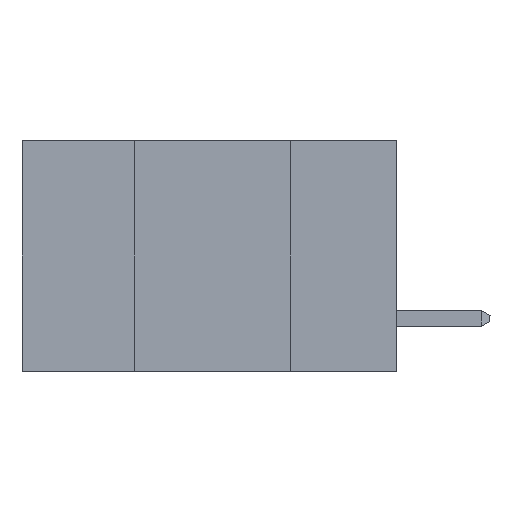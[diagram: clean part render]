
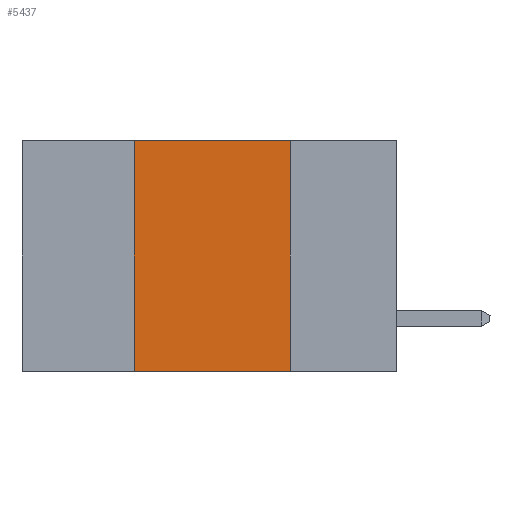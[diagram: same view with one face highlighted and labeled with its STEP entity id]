
A CAD part, left-side view. The second image highlights one B-rep face of the part: STEP entity #5437.
In plain terms, the highlighted planar face has unit normal (-1, 0, 0).
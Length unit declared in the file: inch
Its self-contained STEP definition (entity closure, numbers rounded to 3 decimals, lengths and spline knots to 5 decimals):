
#397 = LINE ( 'NONE', #22797, #23867 ) ;
#603 = DIRECTION ( 'NONE',  ( 0., 0., -1. ) ) ;
#2635 = ORIENTED_EDGE ( 'NONE', *, *, #13744, .F. ) ;
#4188 = LINE ( 'NONE', #6854, #21523 ) ;
#5243 = FACE_OUTER_BOUND ( 'NONE', #16323, .T. ) ;
#5365 = VERTEX_POINT ( 'NONE', #11476 ) ;
#5437 = ADVANCED_FACE ( 'NONE', ( #5243 ), #13830, .F. ) ;
#6231 = DIRECTION ( 'NONE',  ( 0., 0., -1. ) ) ;
#6854 = CARTESIAN_POINT ( 'NONE',  ( 0., 0.6, -0.37 ) ) ;
#8241 = EDGE_CURVE ( 'NONE', #13775, #5365, #397, .T. ) ;
#9029 = VECTOR ( 'NONE', #19841, 39.37008 ) ;
#9602 = LINE ( 'NONE', #14349, #9029 ) ;
#11476 = CARTESIAN_POINT ( 'NONE',  ( 0., 0.17, -0.37 ) ) ;
#11507 = VERTEX_POINT ( 'NONE', #23251 ) ;
#12007 = DIRECTION ( 'NONE',  ( 0., -1., 0. ) ) ;
#13744 = EDGE_CURVE ( 'NONE', #16364, #11507, #14367, .T. ) ;
#13775 = VERTEX_POINT ( 'NONE', #21130 ) ;
#13830 = PLANE ( 'NONE',  #21060 ) ;
#14349 = CARTESIAN_POINT ( 'NONE',  ( 0., 0.6, 0. ) ) ;
#14367 = LINE ( 'NONE', #19155, #18435 ) ;
#15777 = CARTESIAN_POINT ( 'NONE',  ( 0., 0.42, -0.37 ) ) ;
#16323 = EDGE_LOOP ( 'NONE', ( #16845, #18650, #2635, #19335 ) ) ;
#16364 = VERTEX_POINT ( 'NONE', #15777 ) ;
#16845 = ORIENTED_EDGE ( 'NONE', *, *, #8241, .F. ) ;
#17457 = DIRECTION ( 'NONE',  ( 0., 0., 1. ) ) ;
#17958 = EDGE_CURVE ( 'NONE', #16364, #5365, #4188, .T. ) ;
#18435 = VECTOR ( 'NONE', #17457, 39.37008 ) ;
#18650 = ORIENTED_EDGE ( 'NONE', *, *, #23631, .F. ) ;
#19155 = CARTESIAN_POINT ( 'NONE',  ( 0., 0.42, 0. ) ) ;
#19259 = CARTESIAN_POINT ( 'NONE',  ( 0., 0.6, 0. ) ) ;
#19335 = ORIENTED_EDGE ( 'NONE', *, *, #17958, .T. ) ;
#19841 = DIRECTION ( 'NONE',  ( 0., -1., 0. ) ) ;
#21060 = AXIS2_PLACEMENT_3D ( 'NONE', #19259, #21080, #603 ) ;
#21080 = DIRECTION ( 'NONE',  ( 1., 0., 0. ) ) ;
#21130 = CARTESIAN_POINT ( 'NONE',  ( 0., 0.17, 0. ) ) ;
#21523 = VECTOR ( 'NONE', #12007, 39.37008 ) ;
#22797 = CARTESIAN_POINT ( 'NONE',  ( 0., 0.17, 0. ) ) ;
#23251 = CARTESIAN_POINT ( 'NONE',  ( 0., 0.42, 0. ) ) ;
#23631 = EDGE_CURVE ( 'NONE', #11507, #13775, #9602, .T. ) ;
#23867 = VECTOR ( 'NONE', #6231, 39.37008 ) ;
